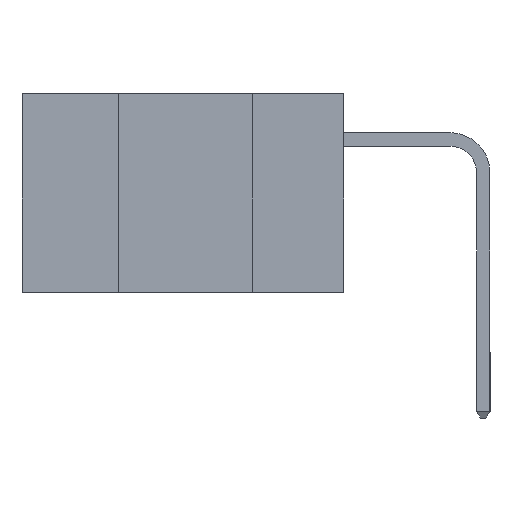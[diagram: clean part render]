
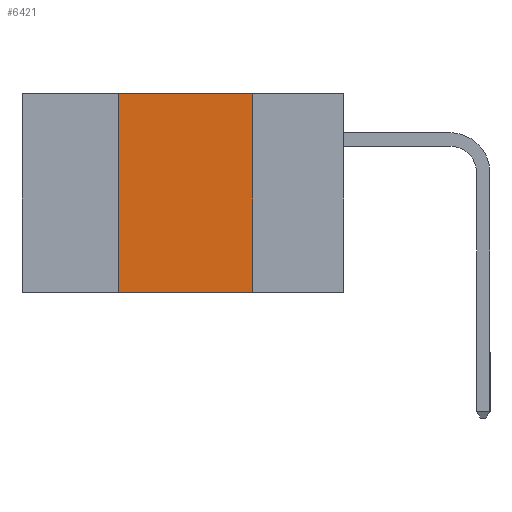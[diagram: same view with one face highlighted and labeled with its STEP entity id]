
A CAD part, left-side view. The second image highlights one B-rep face of the part: STEP entity #6421.
In plain terms, the highlighted planar face has unit normal (-1, 0, 0).
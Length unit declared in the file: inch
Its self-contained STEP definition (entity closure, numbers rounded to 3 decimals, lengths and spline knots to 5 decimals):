
#317 = EDGE_CURVE ( 'NONE', #15503, #2330, #1029, .T. ) ;
#796 = EDGE_CURVE ( 'NONE', #13828, #2330, #1010, .T. ) ;
#1010 = LINE ( 'NONE', #10643, #5049 ) ;
#1029 = LINE ( 'NONE', #11476, #14427 ) ;
#1124 = DIRECTION ( 'NONE',  ( 1., 0., 0. ) ) ;
#1181 = EDGE_CURVE ( 'NONE', #13828, #13915, #8155, .T. ) ;
#1280 = DIRECTION ( 'NONE',  ( 0., -1., 0. ) ) ;
#2330 = VERTEX_POINT ( 'NONE', #7097 ) ;
#3160 = ORIENTED_EDGE ( 'NONE', *, *, #796, .T. ) ;
#3598 = ORIENTED_EDGE ( 'NONE', *, *, #1181, .F. ) ;
#4593 = EDGE_LOOP ( 'NONE', ( #9947, #14817, #3598, #3160 ) ) ;
#5049 = VECTOR ( 'NONE', #1280, 39.37008 ) ;
#6421 = ADVANCED_FACE ( 'NONE', ( #14777 ), #6849, .F. ) ;
#6849 = PLANE ( 'NONE',  #12946 ) ;
#6852 = CARTESIAN_POINT ( 'NONE',  ( 0., 0.42, 0. ) ) ;
#6917 = DIRECTION ( 'NONE',  ( 0., -1., 0. ) ) ;
#7097 = CARTESIAN_POINT ( 'NONE',  ( 0., 0.17, -0.37 ) ) ;
#7255 = CARTESIAN_POINT ( 'NONE',  ( 0., 0.6, 0. ) ) ;
#7918 = EDGE_CURVE ( 'NONE', #13915, #15503, #15298, .T. ) ;
#8155 = LINE ( 'NONE', #14857, #14400 ) ;
#8705 = VECTOR ( 'NONE', #6917, 39.37008 ) ;
#9007 = CARTESIAN_POINT ( 'NONE',  ( 0., 0.17, 0. ) ) ;
#9947 = ORIENTED_EDGE ( 'NONE', *, *, #317, .F. ) ;
#10643 = CARTESIAN_POINT ( 'NONE',  ( 0., 0.6, -0.37 ) ) ;
#10764 = DIRECTION ( 'NONE',  ( 0., 0., 1. ) ) ;
#11476 = CARTESIAN_POINT ( 'NONE',  ( 0., 0.17, 0. ) ) ;
#11942 = DIRECTION ( 'NONE',  ( 0., 0., -1. ) ) ;
#12946 = AXIS2_PLACEMENT_3D ( 'NONE', #7255, #1124, #11942 ) ;
#13828 = VERTEX_POINT ( 'NONE', #16683 ) ;
#13915 = VERTEX_POINT ( 'NONE', #6852 ) ;
#14347 = DIRECTION ( 'NONE',  ( 0., 0., -1. ) ) ;
#14400 = VECTOR ( 'NONE', #10764, 39.37008 ) ;
#14427 = VECTOR ( 'NONE', #14347, 39.37008 ) ;
#14777 = FACE_OUTER_BOUND ( 'NONE', #4593, .T. ) ;
#14817 = ORIENTED_EDGE ( 'NONE', *, *, #7918, .F. ) ;
#14857 = CARTESIAN_POINT ( 'NONE',  ( 0., 0.42, 0. ) ) ;
#15298 = LINE ( 'NONE', #15658, #8705 ) ;
#15503 = VERTEX_POINT ( 'NONE', #9007 ) ;
#15658 = CARTESIAN_POINT ( 'NONE',  ( 0., 0.6, 0. ) ) ;
#16683 = CARTESIAN_POINT ( 'NONE',  ( 0., 0.42, -0.37 ) ) ;
